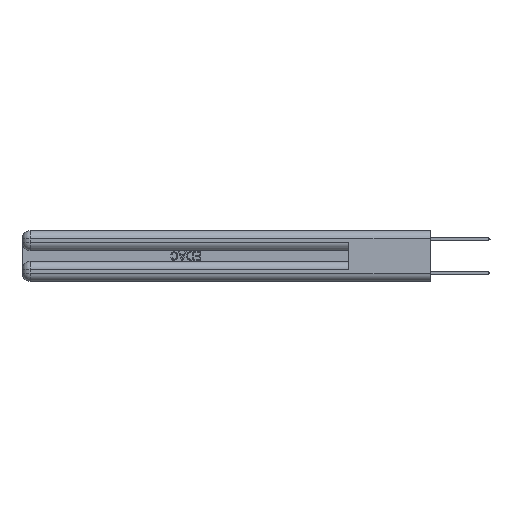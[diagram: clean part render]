
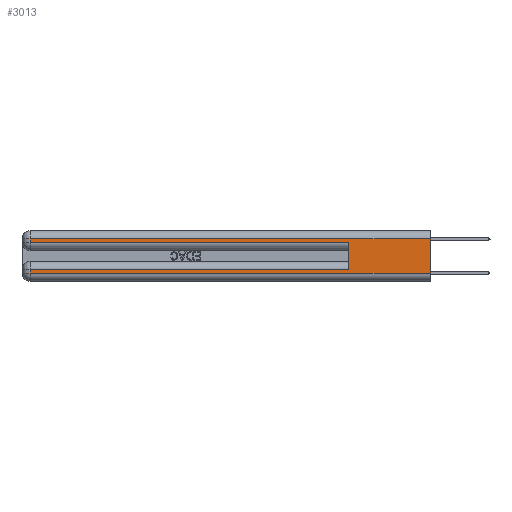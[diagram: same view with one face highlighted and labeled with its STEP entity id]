
A CAD part, left-side view. The second image highlights one B-rep face of the part: STEP entity #3013.
In plain terms, the highlighted planar face has unit normal (-1, 0, 0).
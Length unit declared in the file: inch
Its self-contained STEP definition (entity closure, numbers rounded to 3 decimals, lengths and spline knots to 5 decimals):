
#596 = CARTESIAN_POINT ( 'NONE',  ( 0., 0., 0.06 ) ) ;
#685 = DIRECTION ( 'NONE',  ( 0., -1., 0. ) ) ;
#696 = VERTEX_POINT ( 'NONE', #9339 ) ;
#1049 = EDGE_LOOP ( 'NONE', ( #6316, #5025, #11482, #12974, #1232, #5467, #21794, #9919 ) ) ;
#1232 = ORIENTED_EDGE ( 'NONE', *, *, #9690, .F. ) ;
#1704 = VECTOR ( 'NONE', #14176, 39.37008 ) ;
#1734 = LINE ( 'NONE', #596, #6919 ) ;
#1983 = PLANE ( 'NONE',  #9404 ) ;
#3013 = ADVANCED_FACE ( 'NONE', ( #4835 ), #1983, .F. ) ;
#3076 = CARTESIAN_POINT ( 'NONE',  ( 0., 2.94, 0.06 ) ) ;
#3327 = EDGE_CURVE ( 'NONE', #10493, #12281, #13368, .T. ) ;
#3925 = VERTEX_POINT ( 'NONE', #13540 ) ;
#4188 = VECTOR ( 'NONE', #18246, 39.37008 ) ;
#4519 = LINE ( 'NONE', #27378, #4188 ) ;
#4835 = FACE_OUTER_BOUND ( 'NONE', #1049, .T. ) ;
#5025 = ORIENTED_EDGE ( 'NONE', *, *, #28437, .T. ) ;
#5467 = ORIENTED_EDGE ( 'NONE', *, *, #14658, .T. ) ;
#5636 = CARTESIAN_POINT ( 'NONE',  ( 0., 2.94, 0.285 ) ) ;
#6078 = EDGE_CURVE ( 'NONE', #8948, #19579, #15943, .T. ) ;
#6316 = ORIENTED_EDGE ( 'NONE', *, *, #19517, .F. ) ;
#6428 = DIRECTION ( 'NONE',  ( 0., -1., 0. ) ) ;
#6567 = CARTESIAN_POINT ( 'NONE',  ( 0., 2.94, 0.37 ) ) ;
#6919 = VECTOR ( 'NONE', #685, 39.37008 ) ;
#7541 = VERTEX_POINT ( 'NONE', #22124 ) ;
#7568 = VECTOR ( 'NONE', #6428, 39.37008 ) ;
#7916 = CARTESIAN_POINT ( 'NONE',  ( 0., 0., 0.31 ) ) ;
#8146 = LINE ( 'NONE', #22628, #21456 ) ;
#8948 = VERTEX_POINT ( 'NONE', #20137 ) ;
#9339 = CARTESIAN_POINT ( 'NONE',  ( 0., 0.6, 0.085 ) ) ;
#9404 = AXIS2_PLACEMENT_3D ( 'NONE', #17208, #17307, #12932 ) ;
#9690 = EDGE_CURVE ( 'NONE', #696, #12281, #8146, .T. ) ;
#9762 = LINE ( 'NONE', #6567, #17606 ) ;
#9919 = ORIENTED_EDGE ( 'NONE', *, *, #13729, .T. ) ;
#10493 = VERTEX_POINT ( 'NONE', #5636 ) ;
#10901 = EDGE_CURVE ( 'NONE', #25397, #10493, #9762, .T. ) ;
#10961 = LINE ( 'NONE', #17756, #22581 ) ;
#11482 = ORIENTED_EDGE ( 'NONE', *, *, #10901, .T. ) ;
#12281 = VERTEX_POINT ( 'NONE', #14495 ) ;
#12932 = DIRECTION ( 'NONE',  ( 0., 0., -1. ) ) ;
#12974 = ORIENTED_EDGE ( 'NONE', *, *, #3327, .T. ) ;
#13368 = LINE ( 'NONE', #28102, #7568 ) ;
#13540 = CARTESIAN_POINT ( 'NONE',  ( 0., 0., 0.31 ) ) ;
#13729 = EDGE_CURVE ( 'NONE', #19579, #7541, #1734, .T. ) ;
#14176 = DIRECTION ( 'NONE',  ( 0., 1., 0. ) ) ;
#14495 = CARTESIAN_POINT ( 'NONE',  ( 0., 0.6, 0.285 ) ) ;
#14658 = EDGE_CURVE ( 'NONE', #696, #8948, #10961, .T. ) ;
#15943 = LINE ( 'NONE', #23322, #19763 ) ;
#17208 = CARTESIAN_POINT ( 'NONE',  ( 0., 0., 0.37 ) ) ;
#17307 = DIRECTION ( 'NONE',  ( 1., 0., 0. ) ) ;
#17606 = VECTOR ( 'NONE', #28248, 39.37008 ) ;
#17756 = CARTESIAN_POINT ( 'NONE',  ( 0., 0., 0.085 ) ) ;
#18246 = DIRECTION ( 'NONE',  ( 0., 0., -1. ) ) ;
#19517 = EDGE_CURVE ( 'NONE', #3925, #7541, #4519, .T. ) ;
#19579 = VERTEX_POINT ( 'NONE', #3076 ) ;
#19763 = VECTOR ( 'NONE', #23228, 39.37008 ) ;
#20000 = DIRECTION ( 'NONE',  ( 0., 1., 0. ) ) ;
#20137 = CARTESIAN_POINT ( 'NONE',  ( 0., 2.94, 0.085 ) ) ;
#21456 = VECTOR ( 'NONE', #24868, 39.37008 ) ;
#21794 = ORIENTED_EDGE ( 'NONE', *, *, #6078, .T. ) ;
#22124 = CARTESIAN_POINT ( 'NONE',  ( 0., 0., 0.06 ) ) ;
#22581 = VECTOR ( 'NONE', #20000, 39.37008 ) ;
#22628 = CARTESIAN_POINT ( 'NONE',  ( 0., 0.6, 0.145 ) ) ;
#23228 = DIRECTION ( 'NONE',  ( 0., 0., -1. ) ) ;
#23322 = CARTESIAN_POINT ( 'NONE',  ( 0., 2.94, 0.37 ) ) ;
#24868 = DIRECTION ( 'NONE',  ( 0., 0., 1. ) ) ;
#25065 = LINE ( 'NONE', #7916, #1704 ) ;
#25397 = VERTEX_POINT ( 'NONE', #26949 ) ;
#26949 = CARTESIAN_POINT ( 'NONE',  ( 0., 2.94, 0.31 ) ) ;
#27378 = CARTESIAN_POINT ( 'NONE',  ( 0., 0., 0.37 ) ) ;
#28102 = CARTESIAN_POINT ( 'NONE',  ( 0., 0., 0.285 ) ) ;
#28248 = DIRECTION ( 'NONE',  ( 0., 0., -1. ) ) ;
#28437 = EDGE_CURVE ( 'NONE', #3925, #25397, #25065, .T. ) ;
